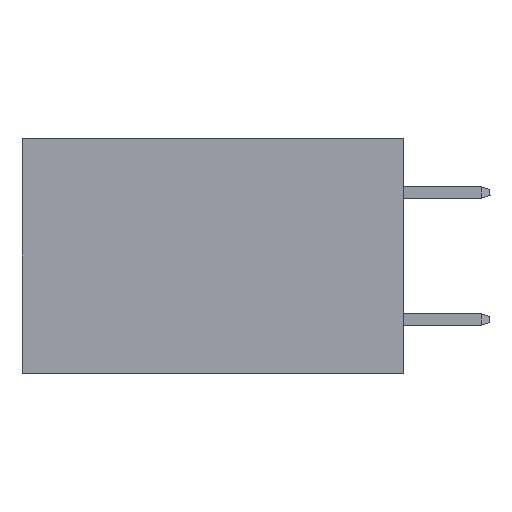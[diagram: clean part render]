
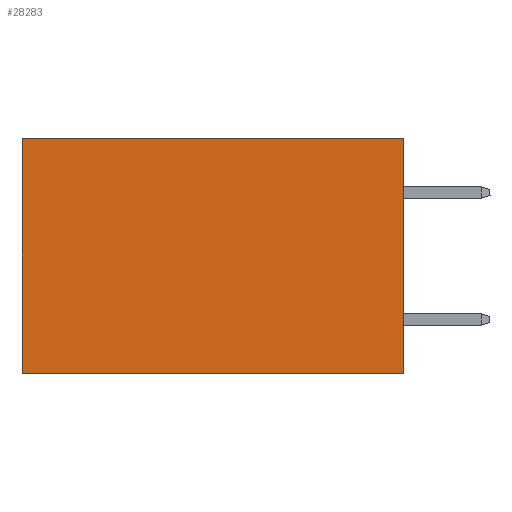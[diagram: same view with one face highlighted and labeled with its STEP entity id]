
A CAD part, left-side view. The second image highlights one B-rep face of the part: STEP entity #28283.
In plain terms, the highlighted planar face has unit normal (-1, 0, 0).
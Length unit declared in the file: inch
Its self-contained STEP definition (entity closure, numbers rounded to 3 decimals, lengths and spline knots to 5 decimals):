
#400 = EDGE_LOOP ( 'NONE', ( #26171, #27734, #42233, #29644 ) ) ;
#452 = LINE ( 'NONE', #39702, #40857 ) ;
#844 = CARTESIAN_POINT ( 'NONE',  ( 0.2875, 0.6, -0.37 ) ) ;
#1511 = LINE ( 'NONE', #36528, #9356 ) ;
#1624 = VERTEX_POINT ( 'NONE', #7926 ) ;
#2417 = EDGE_CURVE ( 'NONE', #2597, #1624, #9658, .T. ) ;
#2597 = VERTEX_POINT ( 'NONE', #37776 ) ;
#3528 = EDGE_CURVE ( 'NONE', #2597, #8879, #452, .T. ) ;
#6034 = FACE_OUTER_BOUND ( 'NONE', #400, .T. ) ;
#7863 = VECTOR ( 'NONE', #23786, 39.37008 ) ;
#7926 = CARTESIAN_POINT ( 'NONE',  ( 0.2875, 0., -0.37 ) ) ;
#8593 = EDGE_CURVE ( 'NONE', #1624, #35112, #45178, .T. ) ;
#8879 = VERTEX_POINT ( 'NONE', #11782 ) ;
#9356 = VECTOR ( 'NONE', #15830, 39.37008 ) ;
#9658 = LINE ( 'NONE', #23555, #7863 ) ;
#11782 = CARTESIAN_POINT ( 'NONE',  ( 0.2875, 0.6, 0. ) ) ;
#12400 = CARTESIAN_POINT ( 'NONE',  ( 0.2875, 0., 0. ) ) ;
#14799 = DIRECTION ( 'NONE',  ( 0., 1., 0. ) ) ;
#15830 = DIRECTION ( 'NONE',  ( 0., 0., -1. ) ) ;
#23555 = CARTESIAN_POINT ( 'NONE',  ( 0.2875, 0., 0. ) ) ;
#23786 = DIRECTION ( 'NONE',  ( 0., 0., -1. ) ) ;
#23812 = CARTESIAN_POINT ( 'NONE',  ( 0.2875, 0., -0.37 ) ) ;
#26171 = ORIENTED_EDGE ( 'NONE', *, *, #40329, .T. ) ;
#27734 = ORIENTED_EDGE ( 'NONE', *, *, #8593, .F. ) ;
#28283 = ADVANCED_FACE ( 'NONE', ( #6034 ), #44367, .F. ) ;
#29644 = ORIENTED_EDGE ( 'NONE', *, *, #3528, .T. ) ;
#34018 = DIRECTION ( 'NONE',  ( 0., 0., -1. ) ) ;
#35112 = VERTEX_POINT ( 'NONE', #844 ) ;
#36528 = CARTESIAN_POINT ( 'NONE',  ( 0.2875, 0.6, 0. ) ) ;
#37329 = DIRECTION ( 'NONE',  ( 1., 0., 0. ) ) ;
#37776 = CARTESIAN_POINT ( 'NONE',  ( 0.2875, 0., 0. ) ) ;
#39702 = CARTESIAN_POINT ( 'NONE',  ( 0.2875, 0., 0. ) ) ;
#40329 = EDGE_CURVE ( 'NONE', #8879, #35112, #1511, .T. ) ;
#40857 = VECTOR ( 'NONE', #14799, 39.37008 ) ;
#41635 = DIRECTION ( 'NONE',  ( 0., 1., 0. ) ) ;
#42233 = ORIENTED_EDGE ( 'NONE', *, *, #2417, .F. ) ;
#44367 = PLANE ( 'NONE',  #46240 ) ;
#45178 = LINE ( 'NONE', #23812, #45879 ) ;
#45879 = VECTOR ( 'NONE', #41635, 39.37008 ) ;
#46240 = AXIS2_PLACEMENT_3D ( 'NONE', #12400, #37329, #34018 ) ;
